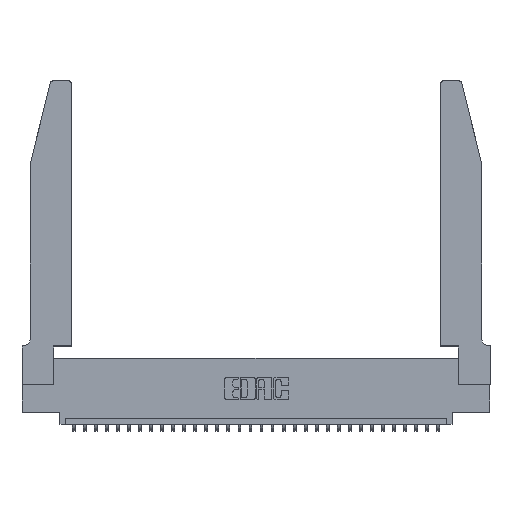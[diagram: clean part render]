
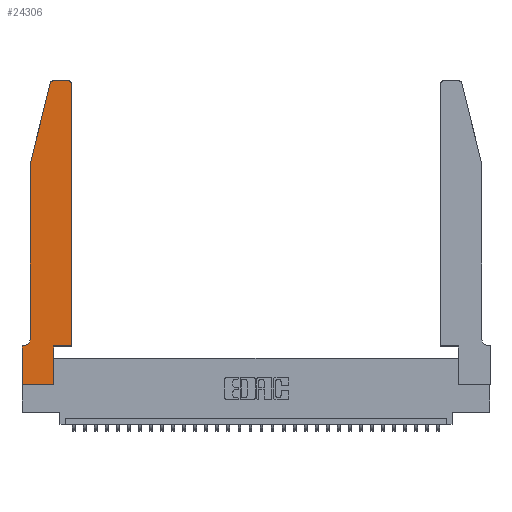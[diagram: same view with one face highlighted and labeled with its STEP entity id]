
A CAD part, top view. The second image highlights one B-rep face of the part: STEP entity #24306.
In plain terms, the highlighted planar face has unit normal (0, 0, 1).
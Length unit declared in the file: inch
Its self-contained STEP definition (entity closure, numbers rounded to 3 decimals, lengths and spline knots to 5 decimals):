
#307 = EDGE_LOOP ( 'NONE', ( #1019, #16570, #22177, #1035, #4357, #24769, #19440, #20551, #15747, #30211, #30645, #13850 ) ) ;
#570 = DIRECTION ( 'NONE',  ( 0., 0., -1. ) ) ;
#725 = CARTESIAN_POINT ( 'NONE',  ( 0., 0., 0.37 ) ) ;
#728 = CARTESIAN_POINT ( 'NONE',  ( 0.4505, 0.35, 0.37 ) ) ;
#787 = CARTESIAN_POINT ( 'NONE',  ( 0., 0.35, 0.37 ) ) ;
#858 = VERTEX_POINT ( 'NONE', #10498 ) ;
#971 = DIRECTION ( 'NONE',  ( 0., 1., 0. ) ) ;
#1019 = ORIENTED_EDGE ( 'NONE', *, *, #9035, .T. ) ;
#1035 = ORIENTED_EDGE ( 'NONE', *, *, #8896, .T. ) ;
#1283 = CARTESIAN_POINT ( 'NONE',  ( 0., 0.35, 0.37 ) ) ;
#2572 = VERTEX_POINT ( 'NONE', #31033 ) ;
#2714 = VERTEX_POINT ( 'NONE', #3541 ) ;
#2789 = DIRECTION ( 'NONE',  ( 0., 0., 1. ) ) ;
#2948 = CIRCLE ( 'NONE', #30210, 0.03 ) ;
#3093 = DIRECTION ( 'NONE',  ( -1., 0., 0. ) ) ;
#3356 = CARTESIAN_POINT ( 'NONE',  ( 0.0755, 0.42, 0.37 ) ) ;
#3540 = VERTEX_POINT ( 'NONE', #6734 ) ;
#3541 = CARTESIAN_POINT ( 'NONE',  ( 0., 0., 0.37 ) ) ;
#3782 = DIRECTION ( 'NONE',  ( -0.239, -0.971, 0. ) ) ;
#4357 = ORIENTED_EDGE ( 'NONE', *, *, #23830, .T. ) ;
#4981 = EDGE_CURVE ( 'NONE', #25069, #2714, #28193, .T. ) ;
#6278 = VERTEX_POINT ( 'NONE', #17693 ) ;
#6734 = CARTESIAN_POINT ( 'NONE',  ( 0.0055, 0.35, 0.37 ) ) ;
#6899 = CARTESIAN_POINT ( 'NONE',  ( 0.4205, 2.72, 0.37 ) ) ;
#7179 = DIRECTION ( 'NONE',  ( 0., 1., 0. ) ) ;
#7532 = DIRECTION ( 'NONE',  ( -1., 0., 0. ) ) ;
#7638 = EDGE_CURVE ( 'NONE', #10938, #858, #18111, .T. ) ;
#8173 = DIRECTION ( 'NONE',  ( 1., 0., 0. ) ) ;
#8406 = CARTESIAN_POINT ( 'NONE',  ( 0.284, 2.75, 0.37 ) ) ;
#8614 = EDGE_CURVE ( 'NONE', #18647, #10938, #27203, .T. ) ;
#8896 = EDGE_CURVE ( 'NONE', #6278, #9026, #26465, .T. ) ;
#9026 = VERTEX_POINT ( 'NONE', #3356 ) ;
#9035 = EDGE_CURVE ( 'NONE', #858, #27384, #12294, .T. ) ;
#9066 = DIRECTION ( 'NONE',  ( 0., -1., 0. ) ) ;
#9230 = VECTOR ( 'NONE', #9066, 39.37008 ) ;
#10498 = CARTESIAN_POINT ( 'NONE',  ( 0.4205, 2.75, 0.37 ) ) ;
#10938 = VERTEX_POINT ( 'NONE', #28900 ) ;
#11182 = VECTOR ( 'NONE', #7532, 39.37008 ) ;
#11358 = CARTESIAN_POINT ( 'NONE',  ( 0., 0., 0.37 ) ) ;
#12294 = LINE ( 'NONE', #18269, #11182 ) ;
#12676 = CARTESIAN_POINT ( 'NONE',  ( 0.0755, 0.35, 0.37 ) ) ;
#12843 = VECTOR ( 'NONE', #28293, 39.37008 ) ;
#13627 = LINE ( 'NONE', #20881, #12843 ) ;
#13850 = ORIENTED_EDGE ( 'NONE', *, *, #7638, .T. ) ;
#14042 = EDGE_CURVE ( 'NONE', #3540, #25069, #21823, .T. ) ;
#14161 = EDGE_CURVE ( 'NONE', #2714, #30505, #16877, .T. ) ;
#14538 = CARTESIAN_POINT ( 'NONE',  ( 0.0755, 2., 0.37 ) ) ;
#14599 = VECTOR ( 'NONE', #971, 39.37008 ) ;
#14833 = AXIS2_PLACEMENT_3D ( 'NONE', #787, #2789, #17898 ) ;
#15545 = CARTESIAN_POINT ( 'NONE',  ( 0.284, 2.72, 0.37 ) ) ;
#15610 = CARTESIAN_POINT ( 'NONE',  ( 0.2865, 0.35, 0.37 ) ) ;
#15747 = ORIENTED_EDGE ( 'NONE', *, *, #31252, .T. ) ;
#16570 = ORIENTED_EDGE ( 'NONE', *, *, #26249, .T. ) ;
#16814 = EDGE_CURVE ( 'NONE', #2572, #6278, #24577, .T. ) ;
#16877 = LINE ( 'NONE', #725, #17266 ) ;
#16888 = LINE ( 'NONE', #15610, #14599 ) ;
#16902 = CARTESIAN_POINT ( 'NONE',  ( 0.4505, 0.35, 0.37 ) ) ;
#17266 = VECTOR ( 'NONE', #20047, 39.37008 ) ;
#17581 = DIRECTION ( 'NONE',  ( -1., 0., 0. ) ) ;
#17693 = CARTESIAN_POINT ( 'NONE',  ( 0.0755, 2., 0.37 ) ) ;
#17898 = DIRECTION ( 'NONE',  ( 1., 0., 0. ) ) ;
#18011 = DIRECTION ( 'NONE',  ( 0., 0., 1. ) ) ;
#18111 = CIRCLE ( 'NONE', #19930, 0.03 ) ;
#18269 = CARTESIAN_POINT ( 'NONE',  ( 0.2605, 2.75, 0.37 ) ) ;
#18435 = CIRCLE ( 'NONE', #24273, 0.07 ) ;
#18647 = VERTEX_POINT ( 'NONE', #728 ) ;
#19440 = ORIENTED_EDGE ( 'NONE', *, *, #4981, .T. ) ;
#19930 = AXIS2_PLACEMENT_3D ( 'NONE', #6899, #24016, #26477 ) ;
#20047 = DIRECTION ( 'NONE',  ( 1., 0., 0. ) ) ;
#20106 = CARTESIAN_POINT ( 'NONE',  ( 0.0055, 0.42, 0.37 ) ) ;
#20252 = FACE_OUTER_BOUND ( 'NONE', #307, .T. ) ;
#20523 = VECTOR ( 'NONE', #28434, 39.37008 ) ;
#20551 = ORIENTED_EDGE ( 'NONE', *, *, #14161, .T. ) ;
#20881 = CARTESIAN_POINT ( 'NONE',  ( 0.4505, 0.35, 0.37 ) ) ;
#21823 = LINE ( 'NONE', #12676, #23388 ) ;
#22177 = ORIENTED_EDGE ( 'NONE', *, *, #16814, .T. ) ;
#23388 = VECTOR ( 'NONE', #17581, 39.37008 ) ;
#23830 = EDGE_CURVE ( 'NONE', #9026, #3540, #18435, .T. ) ;
#24016 = DIRECTION ( 'NONE',  ( 0., 0., 1. ) ) ;
#24273 = AXIS2_PLACEMENT_3D ( 'NONE', #20106, #570, #3093 ) ;
#24306 = ADVANCED_FACE ( 'NONE', ( #20252 ), #27598, .T. ) ;
#24577 = LINE ( 'NONE', #14538, #26484 ) ;
#24769 = ORIENTED_EDGE ( 'NONE', *, *, #14042, .T. ) ;
#25069 = VERTEX_POINT ( 'NONE', #1283 ) ;
#26249 = EDGE_CURVE ( 'NONE', #27384, #2572, #2948, .T. ) ;
#26465 = LINE ( 'NONE', #30313, #9230 ) ;
#26477 = DIRECTION ( 'NONE',  ( 1., 0., 0. ) ) ;
#26484 = VECTOR ( 'NONE', #3782, 39.37008 ) ;
#27080 = CARTESIAN_POINT ( 'NONE',  ( 0.2865, 0., 0.37 ) ) ;
#27203 = LINE ( 'NONE', #16902, #28744 ) ;
#27384 = VERTEX_POINT ( 'NONE', #8406 ) ;
#27585 = EDGE_CURVE ( 'NONE', #30094, #18647, #13627, .T. ) ;
#27598 = PLANE ( 'NONE',  #14833 ) ;
#28193 = LINE ( 'NONE', #11358, #20523 ) ;
#28293 = DIRECTION ( 'NONE',  ( 1., 0., 0. ) ) ;
#28391 = CARTESIAN_POINT ( 'NONE',  ( 0.2865, 0.35, 0.37 ) ) ;
#28434 = DIRECTION ( 'NONE',  ( 0., -1., 0. ) ) ;
#28744 = VECTOR ( 'NONE', #7179, 39.37008 ) ;
#28900 = CARTESIAN_POINT ( 'NONE',  ( 0.4505, 2.72, 0.37 ) ) ;
#30094 = VERTEX_POINT ( 'NONE', #28391 ) ;
#30210 = AXIS2_PLACEMENT_3D ( 'NONE', #15545, #18011, #8173 ) ;
#30211 = ORIENTED_EDGE ( 'NONE', *, *, #27585, .T. ) ;
#30313 = CARTESIAN_POINT ( 'NONE',  ( 0.0755, 2., 0.37 ) ) ;
#30505 = VERTEX_POINT ( 'NONE', #27080 ) ;
#30645 = ORIENTED_EDGE ( 'NONE', *, *, #8614, .T. ) ;
#31033 = CARTESIAN_POINT ( 'NONE',  ( 0.25487, 2.72718, 0.37 ) ) ;
#31252 = EDGE_CURVE ( 'NONE', #30505, #30094, #16888, .T. ) ;
